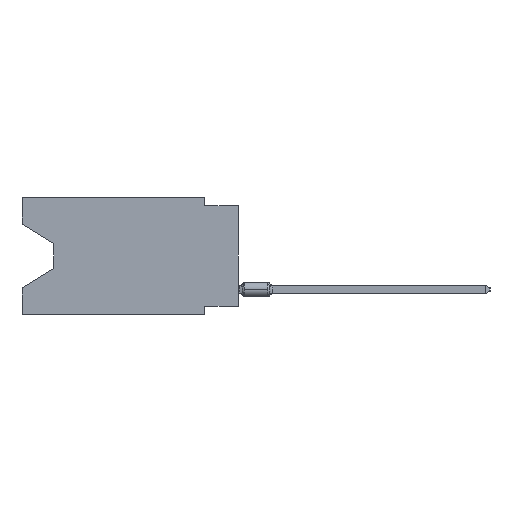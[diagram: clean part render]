
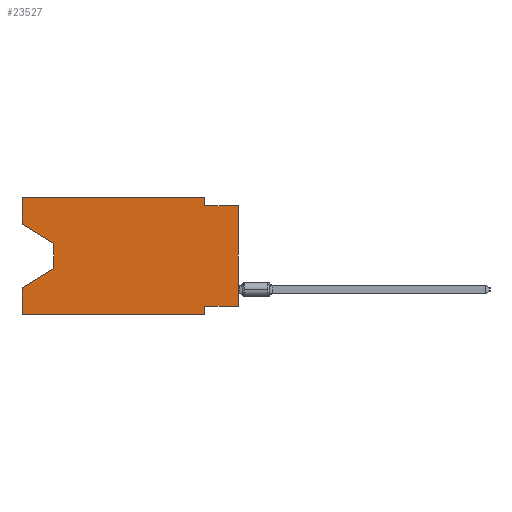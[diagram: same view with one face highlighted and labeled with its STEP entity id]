
A CAD part, left-side view. The second image highlights one B-rep face of the part: STEP entity #23527.
In plain terms, the highlighted planar face has unit normal (-1, 0, 0).
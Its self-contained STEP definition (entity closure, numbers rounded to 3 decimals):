
#2588 = DIRECTION ( 'NONE',  ( 0., 1., 0. ) ) ;
#2636 = CARTESIAN_POINT ( 'NONE',  ( 0., 16.383, -2.038 ) ) ;
#3337 = VECTOR ( 'NONE', #27590, 1000. ) ;
#5271 = CARTESIAN_POINT ( 'NONE',  ( 0., 16.383, 0. ) ) ;
#7245 = CARTESIAN_POINT ( 'NONE',  ( 0., 2.54, -8.89 ) ) ;
#8926 = VECTOR ( 'NONE', #16668, 1000. ) ;
#10034 = DIRECTION ( 'NONE',  ( 0., -1., 0. ) ) ;
#11343 = EDGE_CURVE ( 'NONE', #62078, #24662, #47662, .T. ) ;
#11366 = CARTESIAN_POINT ( 'NONE',  ( 0., 16.383, -8.89 ) ) ;
#13602 = EDGE_CURVE ( 'NONE', #19624, #46550, #62447, .T. ) ;
#14766 = LINE ( 'NONE', #37105, #37101 ) ;
#14852 = VECTOR ( 'NONE', #35409, 1000. ) ;
#14853 = ORIENTED_EDGE ( 'NONE', *, *, #61644, .T. ) ;
#14875 = CARTESIAN_POINT ( 'NONE',  ( 0., 0., 0. ) ) ;
#15654 = CARTESIAN_POINT ( 'NONE',  ( 0., 0., -0.635 ) ) ;
#15832 = DIRECTION ( 'NONE',  ( 0., 0., -1. ) ) ;
#16037 = EDGE_CURVE ( 'NONE', #55990, #46550, #48858, .T. ) ;
#16097 = ORIENTED_EDGE ( 'NONE', *, *, #16037, .F. ) ;
#16177 = ORIENTED_EDGE ( 'NONE', *, *, #46435, .F. ) ;
#16668 = DIRECTION ( 'NONE',  ( 0., 0., 1. ) ) ;
#17653 = AXIS2_PLACEMENT_3D ( 'NONE', #61649, #28682, #40391 ) ;
#17764 = VERTEX_POINT ( 'NONE', #41040 ) ;
#17897 = VERTEX_POINT ( 'NONE', #48338 ) ;
#18043 = CARTESIAN_POINT ( 'NONE',  ( 0., 16.383, -6.852 ) ) ;
#18142 = DIRECTION ( 'NONE',  ( 0., 0., 1. ) ) ;
#19234 = VECTOR ( 'NONE', #15832, 1000. ) ;
#19396 = CARTESIAN_POINT ( 'NONE',  ( 0., 2.54, -8.255 ) ) ;
#19624 = VERTEX_POINT ( 'NONE', #55571 ) ;
#19834 = CARTESIAN_POINT ( 'NONE',  ( 0., 0., -0.635 ) ) ;
#21027 = DIRECTION ( 'NONE',  ( 0., 0., -1. ) ) ;
#21396 = CARTESIAN_POINT ( 'NONE',  ( 0., 13.97, -3.505 ) ) ;
#23445 = VERTEX_POINT ( 'NONE', #21396 ) ;
#23527 = ADVANCED_FACE ( 'NONE', ( #56150 ), #27595, .F. ) ;
#24507 = VECTOR ( 'NONE', #10034, 1000. ) ;
#24593 = LINE ( 'NONE', #2636, #67375 ) ;
#24662 = VERTEX_POINT ( 'NONE', #15654 ) ;
#27467 = CARTESIAN_POINT ( 'NONE',  ( 0., 0., -8.255 ) ) ;
#27590 = DIRECTION ( 'NONE',  ( 0., 0., 1. ) ) ;
#27595 = PLANE ( 'NONE',  #17653 ) ;
#28682 = DIRECTION ( 'NONE',  ( 1., 0., 0. ) ) ;
#33012 = CARTESIAN_POINT ( 'NONE',  ( 0., 13.97, -3.505 ) ) ;
#33401 = CARTESIAN_POINT ( 'NONE',  ( 0., 2.54, 0. ) ) ;
#33883 = DIRECTION ( 'NONE',  ( 0., 0.855, -0.519 ) ) ;
#33904 = VERTEX_POINT ( 'NONE', #57416 ) ;
#34246 = CARTESIAN_POINT ( 'NONE',  ( 0., 13.97, -5.385 ) ) ;
#35409 = DIRECTION ( 'NONE',  ( 0., 0., -1. ) ) ;
#36299 = DIRECTION ( 'NONE',  ( 0., -0.855, -0.519 ) ) ;
#36360 = ORIENTED_EDGE ( 'NONE', *, *, #13602, .T. ) ;
#36858 = EDGE_LOOP ( 'NONE', ( #14853, #42760, #36360, #16097, #52481, #49608, #45624, #61210, #57413, #16177, #57528, #44671 ) ) ;
#37101 = VECTOR ( 'NONE', #37449, 1000. ) ;
#37105 = CARTESIAN_POINT ( 'NONE',  ( 0., 16.383, 0. ) ) ;
#37149 = CARTESIAN_POINT ( 'NONE',  ( 0., 2.54, 0. ) ) ;
#37449 = DIRECTION ( 'NONE',  ( 0., -1., 0. ) ) ;
#38126 = EDGE_CURVE ( 'NONE', #43579, #17764, #57750, .T. ) ;
#39238 = EDGE_CURVE ( 'NONE', #33904, #17897, #45957, .T. ) ;
#39682 = EDGE_CURVE ( 'NONE', #61858, #43579, #69580, .T. ) ;
#40391 = DIRECTION ( 'NONE',  ( 0., 0., -1. ) ) ;
#40469 = VECTOR ( 'NONE', #33883, 1000. ) ;
#41040 = CARTESIAN_POINT ( 'NONE',  ( 0., 2.54, -8.89 ) ) ;
#42257 = CARTESIAN_POINT ( 'NONE',  ( 0., 16.383, -8.89 ) ) ;
#42692 = LINE ( 'NONE', #14875, #8926 ) ;
#42760 = ORIENTED_EDGE ( 'NONE', *, *, #66558, .T. ) ;
#43579 = VERTEX_POINT ( 'NONE', #19396 ) ;
#44671 = ORIENTED_EDGE ( 'NONE', *, *, #39238, .F. ) ;
#45624 = ORIENTED_EDGE ( 'NONE', *, *, #39682, .F. ) ;
#45957 = LINE ( 'NONE', #50383, #64090 ) ;
#46435 = EDGE_CURVE ( 'NONE', #57106, #62078, #71195, .T. ) ;
#46550 = VERTEX_POINT ( 'NONE', #18043 ) ;
#46566 = VECTOR ( 'NONE', #2588, 1000. ) ;
#47662 = LINE ( 'NONE', #19834, #56799 ) ;
#48338 = CARTESIAN_POINT ( 'NONE',  ( 0., 16.383, 0. ) ) ;
#48467 = LINE ( 'NONE', #42257, #24507 ) ;
#48858 = LINE ( 'NONE', #5271, #3337 ) ;
#49511 = LINE ( 'NONE', #33012, #19234 ) ;
#49608 = ORIENTED_EDGE ( 'NONE', *, *, #38126, .F. ) ;
#50383 = CARTESIAN_POINT ( 'NONE',  ( 0., 16.383, 0. ) ) ;
#50586 = EDGE_CURVE ( 'NONE', #61858, #24662, #42692, .T. ) ;
#52436 = DIRECTION ( 'NONE',  ( 0., -1., 0. ) ) ;
#52481 = ORIENTED_EDGE ( 'NONE', *, *, #72182, .T. ) ;
#55571 = CARTESIAN_POINT ( 'NONE',  ( 0., 13.97, -5.385 ) ) ;
#55990 = VERTEX_POINT ( 'NONE', #11366 ) ;
#56150 = FACE_OUTER_BOUND ( 'NONE', #36858, .T. ) ;
#56799 = VECTOR ( 'NONE', #52436, 1000. ) ;
#57106 = VERTEX_POINT ( 'NONE', #33401 ) ;
#57413 = ORIENTED_EDGE ( 'NONE', *, *, #11343, .F. ) ;
#57416 = CARTESIAN_POINT ( 'NONE',  ( 0., 16.383, -2.038 ) ) ;
#57528 = ORIENTED_EDGE ( 'NONE', *, *, #69812, .F. ) ;
#57750 = LINE ( 'NONE', #7245, #14852 ) ;
#61210 = ORIENTED_EDGE ( 'NONE', *, *, #50586, .T. ) ;
#61644 = EDGE_CURVE ( 'NONE', #33904, #23445, #24593, .T. ) ;
#61649 = CARTESIAN_POINT ( 'NONE',  ( 0., 16.383, 0. ) ) ;
#61858 = VERTEX_POINT ( 'NONE', #27467 ) ;
#62078 = VERTEX_POINT ( 'NONE', #63688 ) ;
#62321 = VECTOR ( 'NONE', #21027, 1000. ) ;
#62447 = LINE ( 'NONE', #34246, #40469 ) ;
#63688 = CARTESIAN_POINT ( 'NONE',  ( 0., 2.54, -0.635 ) ) ;
#64090 = VECTOR ( 'NONE', #18142, 1000. ) ;
#66558 = EDGE_CURVE ( 'NONE', #23445, #19624, #49511, .T. ) ;
#67375 = VECTOR ( 'NONE', #36299, 1000. ) ;
#68499 = CARTESIAN_POINT ( 'NONE',  ( 0., 0., -8.255 ) ) ;
#69580 = LINE ( 'NONE', #68499, #46566 ) ;
#69812 = EDGE_CURVE ( 'NONE', #17897, #57106, #14766, .T. ) ;
#71195 = LINE ( 'NONE', #37149, #62321 ) ;
#72182 = EDGE_CURVE ( 'NONE', #55990, #17764, #48467, .T. ) ;
